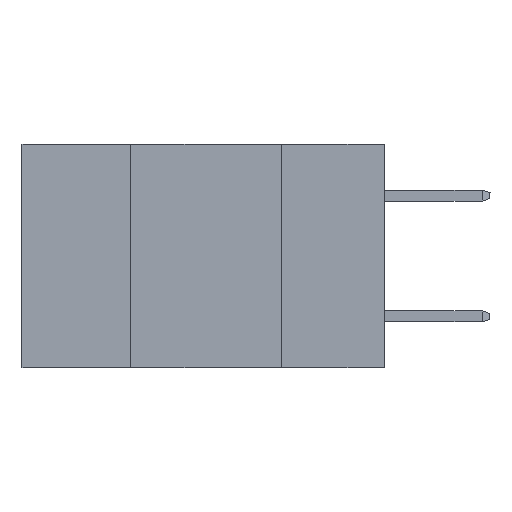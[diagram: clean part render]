
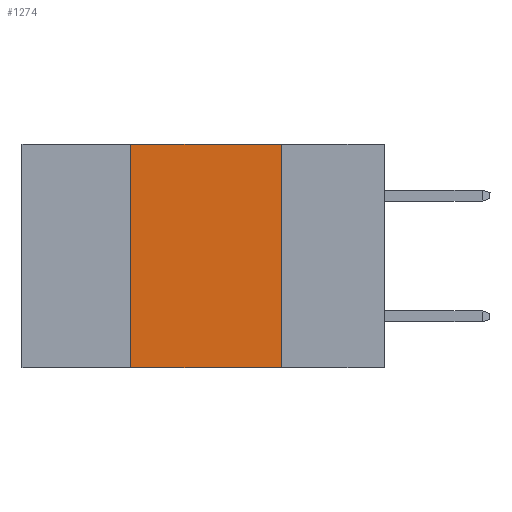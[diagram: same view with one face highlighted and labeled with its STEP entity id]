
A CAD part, left-side view. The second image highlights one B-rep face of the part: STEP entity #1274.
In plain terms, the highlighted planar face has unit normal (-1, 0, 0).
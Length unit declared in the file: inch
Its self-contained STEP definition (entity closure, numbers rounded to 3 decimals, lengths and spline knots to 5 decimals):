
#404 = LINE ( 'NONE', #2879, #5124 ) ;
#442 = VERTEX_POINT ( 'NONE', #4484 ) ;
#674 = CARTESIAN_POINT ( 'NONE',  ( 0., 0.42, -0.37 ) ) ;
#1221 = CARTESIAN_POINT ( 'NONE',  ( 0., 0.42, 0. ) ) ;
#1274 = ADVANCED_FACE ( 'NONE', ( #6837 ), #6645, .F. ) ;
#1644 = CARTESIAN_POINT ( 'NONE',  ( 0., 0.17, 0. ) ) ;
#2033 = DIRECTION ( 'NONE',  ( 0., 0., 1. ) ) ;
#2106 = CARTESIAN_POINT ( 'NONE',  ( 0., 0.6, 0. ) ) ;
#2165 = AXIS2_PLACEMENT_3D ( 'NONE', #3007, #9064, #6810 ) ;
#2383 = EDGE_CURVE ( 'NONE', #442, #3033, #4126, .T. ) ;
#2604 = ORIENTED_EDGE ( 'NONE', *, *, #5728, .F. ) ;
#2879 = CARTESIAN_POINT ( 'NONE',  ( 0., 0.6, -0.37 ) ) ;
#3007 = CARTESIAN_POINT ( 'NONE',  ( 0., 0.6, 0. ) ) ;
#3033 = VERTEX_POINT ( 'NONE', #5544 ) ;
#3299 = LINE ( 'NONE', #2106, #8017 ) ;
#3565 = VERTEX_POINT ( 'NONE', #674 ) ;
#4126 = LINE ( 'NONE', #1644, #9528 ) ;
#4484 = CARTESIAN_POINT ( 'NONE',  ( 0., 0.17, 0. ) ) ;
#4530 = DIRECTION ( 'NONE',  ( 0., -1., 0. ) ) ;
#5124 = VECTOR ( 'NONE', #4530, 39.37008 ) ;
#5294 = EDGE_CURVE ( 'NONE', #3565, #8714, #9394, .T. ) ;
#5544 = CARTESIAN_POINT ( 'NONE',  ( 0., 0.17, -0.37 ) ) ;
#5728 = EDGE_CURVE ( 'NONE', #8714, #442, #3299, .T. ) ;
#6501 = EDGE_CURVE ( 'NONE', #3565, #3033, #404, .T. ) ;
#6645 = PLANE ( 'NONE',  #2165 ) ;
#6720 = CARTESIAN_POINT ( 'NONE',  ( 0., 0.42, 0. ) ) ;
#6810 = DIRECTION ( 'NONE',  ( 0., 0., -1. ) ) ;
#6837 = FACE_OUTER_BOUND ( 'NONE', #8893, .T. ) ;
#7390 = ORIENTED_EDGE ( 'NONE', *, *, #5294, .F. ) ;
#7454 = VECTOR ( 'NONE', #2033, 39.37008 ) ;
#7695 = ORIENTED_EDGE ( 'NONE', *, *, #2383, .F. ) ;
#7985 = ORIENTED_EDGE ( 'NONE', *, *, #6501, .T. ) ;
#8017 = VECTOR ( 'NONE', #8051, 39.37008 ) ;
#8051 = DIRECTION ( 'NONE',  ( 0., -1., 0. ) ) ;
#8173 = DIRECTION ( 'NONE',  ( 0., 0., -1. ) ) ;
#8714 = VERTEX_POINT ( 'NONE', #6720 ) ;
#8893 = EDGE_LOOP ( 'NONE', ( #7695, #2604, #7390, #7985 ) ) ;
#9064 = DIRECTION ( 'NONE',  ( 1., 0., 0. ) ) ;
#9394 = LINE ( 'NONE', #1221, #7454 ) ;
#9528 = VECTOR ( 'NONE', #8173, 39.37008 ) ;
